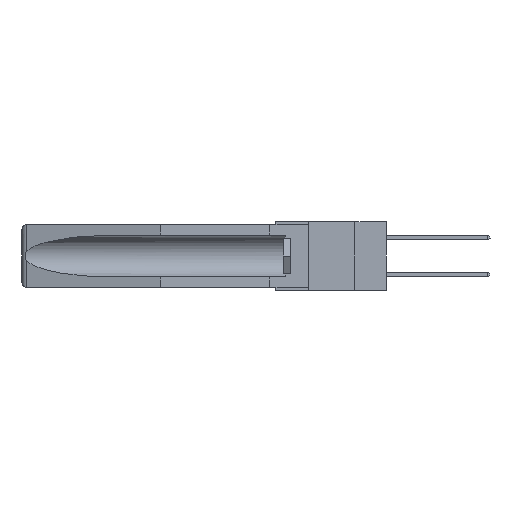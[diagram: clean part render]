
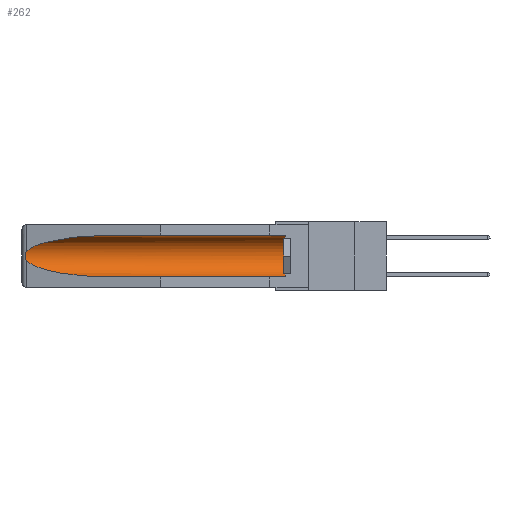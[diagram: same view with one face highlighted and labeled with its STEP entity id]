
A CAD part, left-side view. The second image highlights one B-rep face of the part: STEP entity #262.
In plain terms, the highlighted cylindrical face has radius 2.857 mm (diameter 5.715 mm), a partial arc.
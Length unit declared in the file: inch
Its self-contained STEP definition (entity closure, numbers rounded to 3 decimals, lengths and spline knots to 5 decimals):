
#262 = ADVANCED_FACE ( 'NONE', ( #12568 ), #19568, .F. ) ;
#629 = CARTESIAN_POINT ( 'NONE',  ( 0.2675, 1.53308, -0.16763 ) ) ;
#849 = CARTESIAN_POINT ( 'NONE',  ( 0.26655, 1.53094, -0.18657 ) ) ;
#974 = EDGE_CURVE ( 'NONE', #10497, #18077, #11053, .T. ) ;
#1194 = EDGE_CURVE ( 'NONE', #7281, #18077, #14811, .T. ) ;
#1543 = AXIS2_PLACEMENT_3D ( 'NONE', #11275, #14903, #9285 ) ;
#1574 = ORIENTED_EDGE ( 'NONE', *, *, #15579, .T. ) ;
#1838 = CARTESIAN_POINT ( 'NONE',  ( 0.155, 0.126, -0.284 ) ) ;
#2489 = CARTESIAN_POINT ( 'NONE',  ( 0.25451, 1.48313, -0.09465 ) ) ;
#2840 = AXIS2_PLACEMENT_3D ( 'NONE', #16185, #18051, #12510 ) ;
#3174 = CARTESIAN_POINT ( 'NONE',  ( 0.26537, 1.52718, -0.19328 ) ) ;
#3562 =( BOUNDED_CURVE ( )  B_SPLINE_CURVE ( 3, ( #13950, #21132, #2489, #19484 ),
 .UNSPECIFIED., .F., .F. ) 
 B_SPLINE_CURVE_WITH_KNOTS ( ( 4, 4 ),
 ( 4.71239, 6.08839 ),
 .UNSPECIFIED. ) 
 CURVE ( )  GEOMETRIC_REPRESENTATION_ITEM ( )  RATIONAL_B_SPLINE_CURVE ( ( 1., 0.848, 0.848, 1. ) ) 
 REPRESENTATION_ITEM ( '' )  );
#4271 = B_SPLINE_CURVE_WITH_KNOTS ( 'NONE', 3,
 ( #17745, #23161, #13698, #11803, #629, #4514, #10144, #849, #4591, #6477 ),
 .UNSPECIFIED., .F., .F.,
 ( 4, 2, 2, 2, 4 ),
 ( 0., 0.00029, 0.00058, 0.00087, 0.00117 ),
 .UNSPECIFIED. ) ;
#4514 = CARTESIAN_POINT ( 'NONE',  ( 0.2675, 1.53308, -0.17534 ) ) ;
#4591 = CARTESIAN_POINT ( 'NONE',  ( 0.26597, 1.5296, -0.19026 ) ) ;
#4618 = VECTOR ( 'NONE', #20042, 39.37008 ) ;
#6477 = CARTESIAN_POINT ( 'NONE',  ( 0.26537, 1.52718, -0.19328 ) ) ;
#7281 = VERTEX_POINT ( 'NONE', #3174 ) ;
#7504 = CARTESIAN_POINT ( 'NONE',  ( 0.155, -0.30754, -0.059 ) ) ;
#7872 = VECTOR ( 'NONE', #16822, 39.37008 ) ;
#8928 = ORIENTED_EDGE ( 'NONE', *, *, #10042, .T. ) ;
#9098 = ORIENTED_EDGE ( 'NONE', *, *, #974, .F. ) ;
#9285 = DIRECTION ( 'NONE',  ( 0., 0., 1. ) ) ;
#9839 = VERTEX_POINT ( 'NONE', #15417 ) ;
#10042 = EDGE_CURVE ( 'NONE', #19353, #23688, #3562, .T. ) ;
#10144 = CARTESIAN_POINT ( 'NONE',  ( 0.2673, 1.53269, -0.17917 ) ) ;
#10497 = VERTEX_POINT ( 'NONE', #1838 ) ;
#11053 = LINE ( 'NONE', #23578, #4618 ) ;
#11275 = CARTESIAN_POINT ( 'NONE',  ( 0.155, -0.30754, -0.1715 ) ) ;
#11803 = CARTESIAN_POINT ( 'NONE',  ( 0.2673, 1.5327, -0.16383 ) ) ;
#12278 = CARTESIAN_POINT ( 'NONE',  ( 0.155, 1.07973, -0.284 ) ) ;
#12362 = CARTESIAN_POINT ( 'NONE',  ( 0.21114, 1.30732, -0.284 ) ) ;
#12510 = DIRECTION ( 'NONE',  ( 0., 0., 1. ) ) ;
#12568 = FACE_OUTER_BOUND ( 'NONE', #13303, .T. ) ;
#12598 = CARTESIAN_POINT ( 'NONE',  ( 0.155, 1.07973, -0.284 ) ) ;
#12954 = EDGE_CURVE ( 'NONE', #23688, #7281, #4271, .T. ) ;
#13303 = EDGE_LOOP ( 'NONE', ( #8928, #17794, #18397, #9098, #1574, #22348 ) ) ;
#13473 = CIRCLE ( 'NONE', #2840, 0.1125 ) ;
#13698 = CARTESIAN_POINT ( 'NONE',  ( 0.26654, 1.53092, -0.15636 ) ) ;
#13950 = CARTESIAN_POINT ( 'NONE',  ( 0.155, 1.07973, -0.059 ) ) ;
#14004 = CARTESIAN_POINT ( 'NONE',  ( 0.26537, 1.52718, -0.19328 ) ) ;
#14811 =( BOUNDED_CURVE ( )  B_SPLINE_CURVE ( 3, ( #14004, #19783, #12362, #12278 ),
 .UNSPECIFIED., .F., .F. ) 
 B_SPLINE_CURVE_WITH_KNOTS ( ( 4, 4 ),
 ( 0.1948, 1.5708 ),
 .UNSPECIFIED. ) 
 CURVE ( )  GEOMETRIC_REPRESENTATION_ITEM ( )  RATIONAL_B_SPLINE_CURVE ( ( 1., 0.848, 0.848, 1. ) ) 
 REPRESENTATION_ITEM ( '' )  );
#14903 = DIRECTION ( 'NONE',  ( 0., 1., 0. ) ) ;
#15417 = CARTESIAN_POINT ( 'NONE',  ( 0.155, 0.126, -0.059 ) ) ;
#15579 = EDGE_CURVE ( 'NONE', #10497, #9839, #13473, .T. ) ;
#16185 = CARTESIAN_POINT ( 'NONE',  ( 0.155, 0.126, -0.1715 ) ) ;
#16322 = EDGE_CURVE ( 'NONE', #9839, #19353, #17809, .T. ) ;
#16822 = DIRECTION ( 'NONE',  ( 0., 1., 0. ) ) ;
#17745 = CARTESIAN_POINT ( 'NONE',  ( 0.26537, 1.52718, -0.14972 ) ) ;
#17794 = ORIENTED_EDGE ( 'NONE', *, *, #12954, .T. ) ;
#17809 = LINE ( 'NONE', #7504, #7872 ) ;
#18051 = DIRECTION ( 'NONE',  ( 0., -1., 0. ) ) ;
#18077 = VERTEX_POINT ( 'NONE', #12598 ) ;
#18397 = ORIENTED_EDGE ( 'NONE', *, *, #1194, .T. ) ;
#19293 = CARTESIAN_POINT ( 'NONE',  ( 0.155, 1.07973, -0.059 ) ) ;
#19353 = VERTEX_POINT ( 'NONE', #19293 ) ;
#19484 = CARTESIAN_POINT ( 'NONE',  ( 0.26537, 1.52718, -0.14972 ) ) ;
#19568 = CYLINDRICAL_SURFACE ( 'NONE', #1543, 0.1125 ) ;
#19783 = CARTESIAN_POINT ( 'NONE',  ( 0.25451, 1.48313, -0.24835 ) ) ;
#20042 = DIRECTION ( 'NONE',  ( 0., 1., 0. ) ) ;
#20466 = CARTESIAN_POINT ( 'NONE',  ( 0.26537, 1.52718, -0.14972 ) ) ;
#21132 = CARTESIAN_POINT ( 'NONE',  ( 0.21114, 1.30732, -0.059 ) ) ;
#22348 = ORIENTED_EDGE ( 'NONE', *, *, #16322, .T. ) ;
#23161 = CARTESIAN_POINT ( 'NONE',  ( 0.26597, 1.52961, -0.15275 ) ) ;
#23578 = CARTESIAN_POINT ( 'NONE',  ( 0.155, -0.30754, -0.284 ) ) ;
#23688 = VERTEX_POINT ( 'NONE', #20466 ) ;
